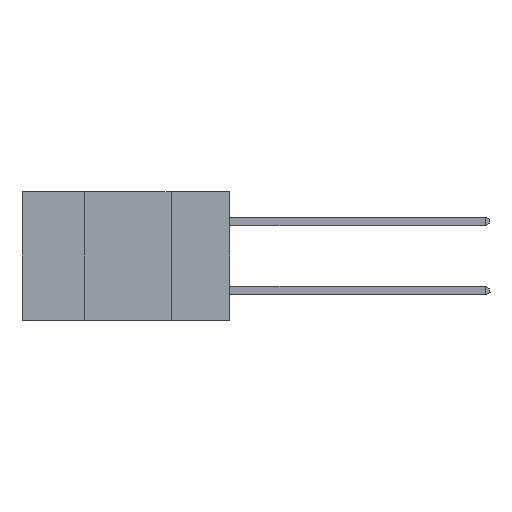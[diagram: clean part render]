
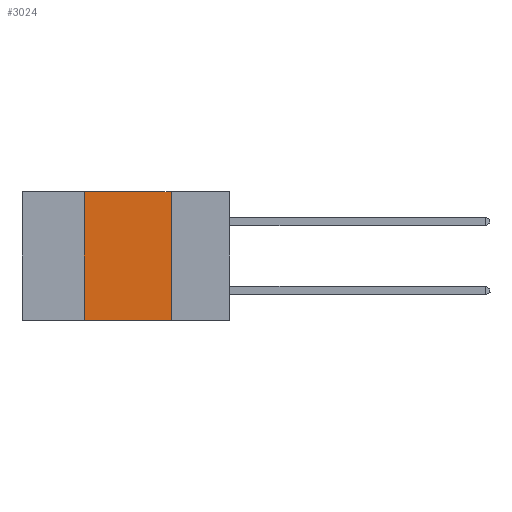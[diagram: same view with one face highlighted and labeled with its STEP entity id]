
A CAD part, left-side view. The second image highlights one B-rep face of the part: STEP entity #3024.
In plain terms, the highlighted planar face has unit normal (-1, 0, 0).
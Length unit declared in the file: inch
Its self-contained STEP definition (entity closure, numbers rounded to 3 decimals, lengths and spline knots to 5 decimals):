
#980 = VERTEX_POINT ( 'NONE', #9989 ) ;
#1130 = ORIENTED_EDGE ( 'NONE', *, *, #2474, .F. ) ;
#1370 = CARTESIAN_POINT ( 'NONE',  ( 0., 0.42, 0. ) ) ;
#1506 = DIRECTION ( 'NONE',  ( 1., 0., 0. ) ) ;
#1596 = CARTESIAN_POINT ( 'NONE',  ( 0., 0.17, 0. ) ) ;
#1967 = ORIENTED_EDGE ( 'NONE', *, *, #11392, .T. ) ;
#2474 = EDGE_CURVE ( 'NONE', #980, #7790, #11131, .T. ) ;
#3024 = ADVANCED_FACE ( 'NONE', ( #8097 ), #4239, .F. ) ;
#3265 = CARTESIAN_POINT ( 'NONE',  ( 0., 0.42, 0. ) ) ;
#3675 = EDGE_CURVE ( 'NONE', #7790, #4935, #11399, .T. ) ;
#4144 = DIRECTION ( 'NONE',  ( 0., -1., 0. ) ) ;
#4191 = EDGE_CURVE ( 'NONE', #4935, #8075, #9393, .T. ) ;
#4239 = PLANE ( 'NONE',  #9459 ) ;
#4488 = CARTESIAN_POINT ( 'NONE',  ( 0., 0.6, 0. ) ) ;
#4511 = VECTOR ( 'NONE', #4999, 39.37008 ) ;
#4920 = CARTESIAN_POINT ( 'NONE',  ( 0., 0.17, 0. ) ) ;
#4935 = VERTEX_POINT ( 'NONE', #1596 ) ;
#4999 = DIRECTION ( 'NONE',  ( 0., 0., -1. ) ) ;
#5177 = CARTESIAN_POINT ( 'NONE',  ( 0., 0.6, 0. ) ) ;
#6055 = LINE ( 'NONE', #10602, #10797 ) ;
#7589 = CARTESIAN_POINT ( 'NONE',  ( 0., 0.17, -0.37 ) ) ;
#7790 = VERTEX_POINT ( 'NONE', #3265 ) ;
#7899 = EDGE_LOOP ( 'NONE', ( #10348, #9053, #1130, #1967 ) ) ;
#8075 = VERTEX_POINT ( 'NONE', #7589 ) ;
#8097 = FACE_OUTER_BOUND ( 'NONE', #7899, .T. ) ;
#8703 = VECTOR ( 'NONE', #10547, 39.37008 ) ;
#9053 = ORIENTED_EDGE ( 'NONE', *, *, #3675, .F. ) ;
#9393 = LINE ( 'NONE', #4920, #4511 ) ;
#9459 = AXIS2_PLACEMENT_3D ( 'NONE', #5177, #1506, #10650 ) ;
#9989 = CARTESIAN_POINT ( 'NONE',  ( 0., 0.42, -0.37 ) ) ;
#10348 = ORIENTED_EDGE ( 'NONE', *, *, #4191, .F. ) ;
#10547 = DIRECTION ( 'NONE',  ( 0., 0., 1. ) ) ;
#10602 = CARTESIAN_POINT ( 'NONE',  ( 0., 0.6, -0.37 ) ) ;
#10650 = DIRECTION ( 'NONE',  ( 0., 0., -1. ) ) ;
#10797 = VECTOR ( 'NONE', #4144, 39.37008 ) ;
#10908 = DIRECTION ( 'NONE',  ( 0., -1., 0. ) ) ;
#11131 = LINE ( 'NONE', #1370, #8703 ) ;
#11392 = EDGE_CURVE ( 'NONE', #980, #8075, #6055, .T. ) ;
#11399 = LINE ( 'NONE', #4488, #11681 ) ;
#11681 = VECTOR ( 'NONE', #10908, 39.37008 ) ;
